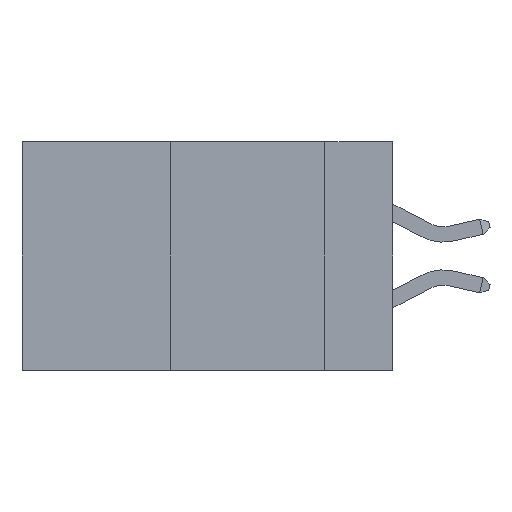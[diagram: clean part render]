
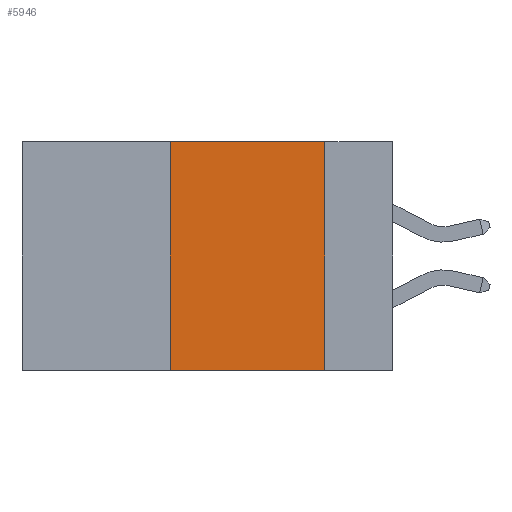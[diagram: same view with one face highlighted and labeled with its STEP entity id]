
A CAD part, left-side view. The second image highlights one B-rep face of the part: STEP entity #5946.
In plain terms, the highlighted planar face has unit normal (-1, 0, 0).
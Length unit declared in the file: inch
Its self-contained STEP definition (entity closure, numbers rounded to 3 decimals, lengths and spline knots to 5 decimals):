
#2074 = ORIENTED_EDGE ( 'NONE', *, *, #19423, .T. ) ;
#2159 = EDGE_CURVE ( 'NONE', #32733, #24189, #13440, .T. ) ;
#3399 = CARTESIAN_POINT ( 'NONE',  ( 0., 0.11, 0. ) ) ;
#4085 = DIRECTION ( 'NONE',  ( 0., -1., 0. ) ) ;
#4109 = EDGE_CURVE ( 'NONE', #11319, #21260, #33451, .T. ) ;
#4928 = VECTOR ( 'NONE', #6595, 39.37008 ) ;
#5533 = VECTOR ( 'NONE', #9736, 39.37008 ) ;
#5946 = ADVANCED_FACE ( 'NONE', ( #23476 ), #31193, .F. ) ;
#6487 = VECTOR ( 'NONE', #18096, 39.37008 ) ;
#6595 = DIRECTION ( 'NONE',  ( 0., -1., 0. ) ) ;
#6768 = CARTESIAN_POINT ( 'NONE',  ( 0., 0.11, 0. ) ) ;
#7092 = VECTOR ( 'NONE', #4085, 39.37008 ) ;
#9736 = DIRECTION ( 'NONE',  ( 0., 0., 1. ) ) ;
#10292 = DIRECTION ( 'NONE',  ( 1., 0., 0. ) ) ;
#10736 = AXIS2_PLACEMENT_3D ( 'NONE', #13037, #10292, #18190 ) ;
#11319 = VERTEX_POINT ( 'NONE', #21389 ) ;
#12721 = LINE ( 'NONE', #27590, #4928 ) ;
#13037 = CARTESIAN_POINT ( 'NONE',  ( 0., 0.6, 0. ) ) ;
#13440 = LINE ( 'NONE', #6768, #6487 ) ;
#14572 = CARTESIAN_POINT ( 'NONE',  ( 0., 0.36, 0. ) ) ;
#17642 = ORIENTED_EDGE ( 'NONE', *, *, #4109, .F. ) ;
#18096 = DIRECTION ( 'NONE',  ( 0., 0., -1. ) ) ;
#18190 = DIRECTION ( 'NONE',  ( 0., 0., -1. ) ) ;
#18656 = ORIENTED_EDGE ( 'NONE', *, *, #26093, .F. ) ;
#19423 = EDGE_CURVE ( 'NONE', #11319, #24189, #32918, .T. ) ;
#20391 = CARTESIAN_POINT ( 'NONE',  ( 0., 0.11, -0.37 ) ) ;
#21260 = VERTEX_POINT ( 'NONE', #29454 ) ;
#21389 = CARTESIAN_POINT ( 'NONE',  ( 0., 0.36, -0.37 ) ) ;
#22675 = CARTESIAN_POINT ( 'NONE',  ( 0., 0.6, -0.37 ) ) ;
#22879 = EDGE_LOOP ( 'NONE', ( #31298, #18656, #17642, #2074 ) ) ;
#23476 = FACE_OUTER_BOUND ( 'NONE', #22879, .T. ) ;
#24189 = VERTEX_POINT ( 'NONE', #20391 ) ;
#26093 = EDGE_CURVE ( 'NONE', #21260, #32733, #12721, .T. ) ;
#27590 = CARTESIAN_POINT ( 'NONE',  ( 0., 0.6, 0. ) ) ;
#29454 = CARTESIAN_POINT ( 'NONE',  ( 0., 0.36, 0. ) ) ;
#31193 = PLANE ( 'NONE',  #10736 ) ;
#31298 = ORIENTED_EDGE ( 'NONE', *, *, #2159, .F. ) ;
#32733 = VERTEX_POINT ( 'NONE', #3399 ) ;
#32918 = LINE ( 'NONE', #22675, #7092 ) ;
#33451 = LINE ( 'NONE', #14572, #5533 ) ;
